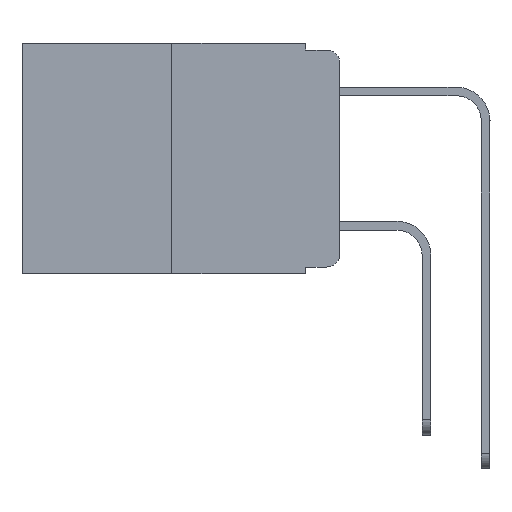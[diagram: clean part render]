
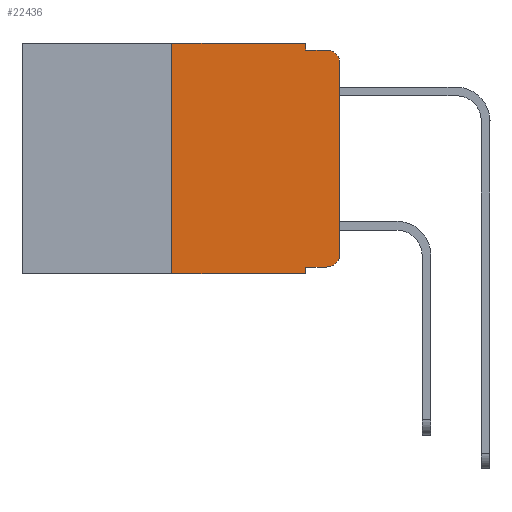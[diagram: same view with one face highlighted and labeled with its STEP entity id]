
A CAD part, left-side view. The second image highlights one B-rep face of the part: STEP entity #22436.
In plain terms, the highlighted planar face has unit normal (-1, 0, 0).
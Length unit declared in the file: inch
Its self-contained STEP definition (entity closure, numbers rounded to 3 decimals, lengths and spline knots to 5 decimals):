
#595 = CARTESIAN_POINT ( 'NONE',  ( 0., 0.25, 0. ) ) ;
#1026 = VECTOR ( 'NONE', #9593, 39.37008 ) ;
#1154 = FACE_OUTER_BOUND ( 'NONE', #17673, .T. ) ;
#1459 = CIRCLE ( 'NONE', #14189, 0.02 ) ;
#1692 = LINE ( 'NONE', #26799, #1026 ) ;
#1850 = AXIS2_PLACEMENT_3D ( 'NONE', #23579, #10673, #25712 ) ;
#2097 = CARTESIAN_POINT ( 'NONE',  ( 0., 0., 0. ) ) ;
#2125 = DIRECTION ( 'NONE',  ( 1., 0., 0. ) ) ;
#2641 = CARTESIAN_POINT ( 'NONE',  ( 0., 0.051, 0. ) ) ;
#2675 = ORIENTED_EDGE ( 'NONE', *, *, #21087, .F. ) ;
#2947 = CARTESIAN_POINT ( 'NONE',  ( 0., 0., -0.03 ) ) ;
#3953 = DIRECTION ( 'NONE',  ( 0., 0., -1. ) ) ;
#4085 = VERTEX_POINT ( 'NONE', #7315 ) ;
#4732 = LINE ( 'NONE', #16257, #9862 ) ;
#4829 = VECTOR ( 'NONE', #7771, 39.37008 ) ;
#5436 = VERTEX_POINT ( 'NONE', #8561 ) ;
#5587 = LINE ( 'NONE', #11754, #22206 ) ;
#5640 = VECTOR ( 'NONE', #3953, 39.37008 ) ;
#5934 = EDGE_CURVE ( 'NONE', #25103, #4085, #1459, .T. ) ;
#5990 = CARTESIAN_POINT ( 'NONE',  ( 0., 0.25, -0.343 ) ) ;
#7234 = LINE ( 'NONE', #2097, #23128 ) ;
#7315 = CARTESIAN_POINT ( 'NONE',  ( 0., 0., -0.313 ) ) ;
#7565 = DIRECTION ( 'NONE',  ( 0., -1., 0. ) ) ;
#7771 = DIRECTION ( 'NONE',  ( 0., -1., 0. ) ) ;
#7858 = VERTEX_POINT ( 'NONE', #2947 ) ;
#7971 = DIRECTION ( 'NONE',  ( -1., 0., 0. ) ) ;
#8512 = ORIENTED_EDGE ( 'NONE', *, *, #10476, .T. ) ;
#8561 = CARTESIAN_POINT ( 'NONE',  ( 0., 0.051, 0. ) ) ;
#8738 = VERTEX_POINT ( 'NONE', #5990 ) ;
#9295 = CARTESIAN_POINT ( 'NONE',  ( 0., 0.051, -0.343 ) ) ;
#9593 = DIRECTION ( 'NONE',  ( 0., -1., 0. ) ) ;
#9862 = VECTOR ( 'NONE', #7565, 39.37008 ) ;
#10476 = EDGE_CURVE ( 'NONE', #8738, #17987, #1692, .T. ) ;
#10673 = DIRECTION ( 'NONE',  ( -1., 0., 0. ) ) ;
#11523 = EDGE_CURVE ( 'NONE', #21236, #17987, #18667, .T. ) ;
#11754 = CARTESIAN_POINT ( 'NONE',  ( 0., 0.473, 0. ) ) ;
#11789 = VERTEX_POINT ( 'NONE', #20885 ) ;
#11874 = CARTESIAN_POINT ( 'NONE',  ( 0., 0.02, -0.01 ) ) ;
#13045 = PLANE ( 'NONE',  #17745 ) ;
#14189 = AXIS2_PLACEMENT_3D ( 'NONE', #20922, #7971, #23101 ) ;
#14432 = EDGE_CURVE ( 'NONE', #7858, #14798, #25582, .T. ) ;
#14798 = VERTEX_POINT ( 'NONE', #11874 ) ;
#15209 = CARTESIAN_POINT ( 'NONE',  ( 0., 0.473, 0. ) ) ;
#16095 = DIRECTION ( 'NONE',  ( 0., -1., 0. ) ) ;
#16238 = CARTESIAN_POINT ( 'NONE',  ( 0., 0.051, -0.333 ) ) ;
#16257 = CARTESIAN_POINT ( 'NONE',  ( 0., 0.051, -0.333 ) ) ;
#16987 = EDGE_CURVE ( 'NONE', #21236, #25103, #4732, .T. ) ;
#17397 = DIRECTION ( 'NONE',  ( 0., 0., -1. ) ) ;
#17673 = EDGE_LOOP ( 'NONE', ( #26693, #28038, #23061, #18674, #24381, #2675, #8512, #26370, #21393, #27716 ) ) ;
#17745 = AXIS2_PLACEMENT_3D ( 'NONE', #15209, #2125, #17397 ) ;
#17876 = DIRECTION ( 'NONE',  ( 0., 0., -1. ) ) ;
#17987 = VERTEX_POINT ( 'NONE', #9295 ) ;
#18056 = DIRECTION ( 'NONE',  ( 0., 0., 1. ) ) ;
#18127 = VECTOR ( 'NONE', #18056, 39.37008 ) ;
#18667 = LINE ( 'NONE', #2641, #19359 ) ;
#18674 = ORIENTED_EDGE ( 'NONE', *, *, #19581, .F. ) ;
#19359 = VECTOR ( 'NONE', #17876, 39.37008 ) ;
#19485 = LINE ( 'NONE', #595, #18127 ) ;
#19581 = EDGE_CURVE ( 'NONE', #5436, #11789, #22922, .T. ) ;
#20478 = EDGE_CURVE ( 'NONE', #25444, #5436, #5587, .T. ) ;
#20885 = CARTESIAN_POINT ( 'NONE',  ( 0., 0.051, -0.01 ) ) ;
#20922 = CARTESIAN_POINT ( 'NONE',  ( 0., 0.02, -0.313 ) ) ;
#21087 = EDGE_CURVE ( 'NONE', #8738, #25444, #19485, .T. ) ;
#21236 = VERTEX_POINT ( 'NONE', #16238 ) ;
#21393 = ORIENTED_EDGE ( 'NONE', *, *, #16987, .T. ) ;
#21455 = LINE ( 'NONE', #22901, #4829 ) ;
#21699 = DIRECTION ( 'NONE',  ( 0., 0., 1. ) ) ;
#21889 = EDGE_CURVE ( 'NONE', #11789, #14798, #21455, .T. ) ;
#22206 = VECTOR ( 'NONE', #16095, 39.37008 ) ;
#22436 = ADVANCED_FACE ( 'NONE', ( #1154 ), #13045, .F. ) ;
#22631 = CARTESIAN_POINT ( 'NONE',  ( 0., 0.02, -0.333 ) ) ;
#22901 = CARTESIAN_POINT ( 'NONE',  ( 0., 0.051, -0.01 ) ) ;
#22922 = LINE ( 'NONE', #27550, #5640 ) ;
#23061 = ORIENTED_EDGE ( 'NONE', *, *, #21889, .F. ) ;
#23101 = DIRECTION ( 'NONE',  ( 0., 0., -1. ) ) ;
#23128 = VECTOR ( 'NONE', #21699, 39.37008 ) ;
#23579 = CARTESIAN_POINT ( 'NONE',  ( 0., 0.02, -0.03 ) ) ;
#24381 = ORIENTED_EDGE ( 'NONE', *, *, #20478, .F. ) ;
#24845 = EDGE_CURVE ( 'NONE', #4085, #7858, #7234, .T. ) ;
#25103 = VERTEX_POINT ( 'NONE', #22631 ) ;
#25444 = VERTEX_POINT ( 'NONE', #25947 ) ;
#25582 = CIRCLE ( 'NONE', #1850, 0.02 ) ;
#25712 = DIRECTION ( 'NONE',  ( 0., 0., -1. ) ) ;
#25947 = CARTESIAN_POINT ( 'NONE',  ( 0., 0.25, 0. ) ) ;
#26370 = ORIENTED_EDGE ( 'NONE', *, *, #11523, .F. ) ;
#26693 = ORIENTED_EDGE ( 'NONE', *, *, #24845, .T. ) ;
#26799 = CARTESIAN_POINT ( 'NONE',  ( 0., 0.473, -0.343 ) ) ;
#27550 = CARTESIAN_POINT ( 'NONE',  ( 0., 0.051, 0. ) ) ;
#27716 = ORIENTED_EDGE ( 'NONE', *, *, #5934, .T. ) ;
#28038 = ORIENTED_EDGE ( 'NONE', *, *, #14432, .T. ) ;
